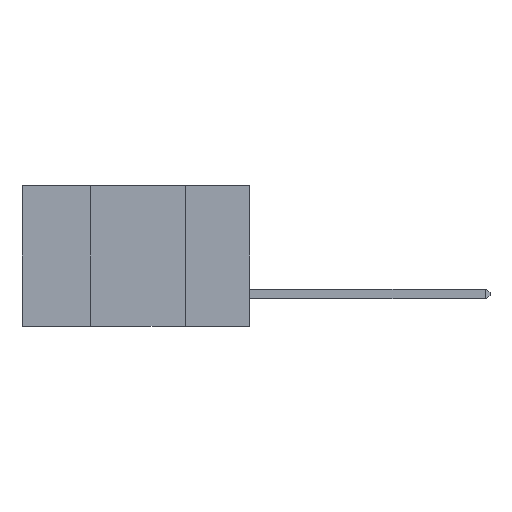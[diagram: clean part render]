
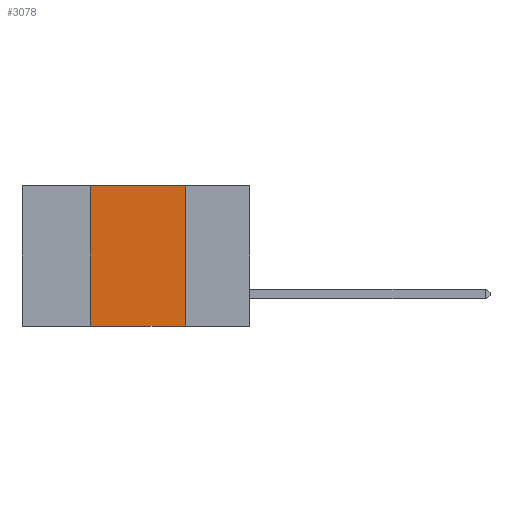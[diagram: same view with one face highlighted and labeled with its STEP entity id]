
A CAD part, left-side view. The second image highlights one B-rep face of the part: STEP entity #3078.
In plain terms, the highlighted planar face has unit normal (-1, 0, 0).
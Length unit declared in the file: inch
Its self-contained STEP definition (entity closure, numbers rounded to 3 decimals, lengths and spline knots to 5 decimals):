
#725 = LINE ( 'NONE', #10105, #5262 ) ;
#867 = CARTESIAN_POINT ( 'NONE',  ( 0., 0.6, 0. ) ) ;
#1034 = VECTOR ( 'NONE', #3065, 39.37008 ) ;
#1043 = EDGE_CURVE ( 'NONE', #3634, #3980, #3194, .T. ) ;
#1060 = EDGE_CURVE ( 'NONE', #8459, #1748, #725, .T. ) ;
#1107 = EDGE_CURVE ( 'NONE', #8459, #3980, #11167, .T. ) ;
#1748 = VERTEX_POINT ( 'NONE', #5548 ) ;
#2082 = VECTOR ( 'NONE', #5483, 39.37008 ) ;
#2341 = EDGE_LOOP ( 'NONE', ( #4390, #9058, #11152, #9310 ) ) ;
#3065 = DIRECTION ( 'NONE',  ( 0., 0., -1. ) ) ;
#3078 = ADVANCED_FACE ( 'NONE', ( #10427 ), #4178, .F. ) ;
#3194 = LINE ( 'NONE', #10244, #1034 ) ;
#3634 = VERTEX_POINT ( 'NONE', #6890 ) ;
#3980 = VERTEX_POINT ( 'NONE', #8659 ) ;
#4016 = DIRECTION ( 'NONE',  ( 0., 0., -1. ) ) ;
#4068 = DIRECTION ( 'NONE',  ( 1., 0., 0. ) ) ;
#4151 = CARTESIAN_POINT ( 'NONE',  ( 0., 0.6, 0. ) ) ;
#4178 = PLANE ( 'NONE',  #5485 ) ;
#4390 = ORIENTED_EDGE ( 'NONE', *, *, #1043, .F. ) ;
#5262 = VECTOR ( 'NONE', #10081, 39.37008 ) ;
#5483 = DIRECTION ( 'NONE',  ( 0., -1., 0. ) ) ;
#5485 = AXIS2_PLACEMENT_3D ( 'NONE', #4151, #4068, #4016 ) ;
#5548 = CARTESIAN_POINT ( 'NONE',  ( 0., 0.42, 0. ) ) ;
#6890 = CARTESIAN_POINT ( 'NONE',  ( 0., 0.17, 0. ) ) ;
#6932 = CARTESIAN_POINT ( 'NONE',  ( 0., 0.42, -0.37 ) ) ;
#6991 = EDGE_CURVE ( 'NONE', #1748, #3634, #7509, .T. ) ;
#7179 = DIRECTION ( 'NONE',  ( 0., -1., 0. ) ) ;
#7234 = VECTOR ( 'NONE', #7179, 39.37008 ) ;
#7509 = LINE ( 'NONE', #867, #7234 ) ;
#8459 = VERTEX_POINT ( 'NONE', #6932 ) ;
#8659 = CARTESIAN_POINT ( 'NONE',  ( 0., 0.17, -0.37 ) ) ;
#9058 = ORIENTED_EDGE ( 'NONE', *, *, #6991, .F. ) ;
#9310 = ORIENTED_EDGE ( 'NONE', *, *, #1107, .T. ) ;
#9431 = CARTESIAN_POINT ( 'NONE',  ( 0., 0.6, -0.37 ) ) ;
#10081 = DIRECTION ( 'NONE',  ( 0., 0., 1. ) ) ;
#10105 = CARTESIAN_POINT ( 'NONE',  ( 0., 0.42, 0. ) ) ;
#10244 = CARTESIAN_POINT ( 'NONE',  ( 0., 0.17, 0. ) ) ;
#10427 = FACE_OUTER_BOUND ( 'NONE', #2341, .T. ) ;
#11152 = ORIENTED_EDGE ( 'NONE', *, *, #1060, .F. ) ;
#11167 = LINE ( 'NONE', #9431, #2082 ) ;
